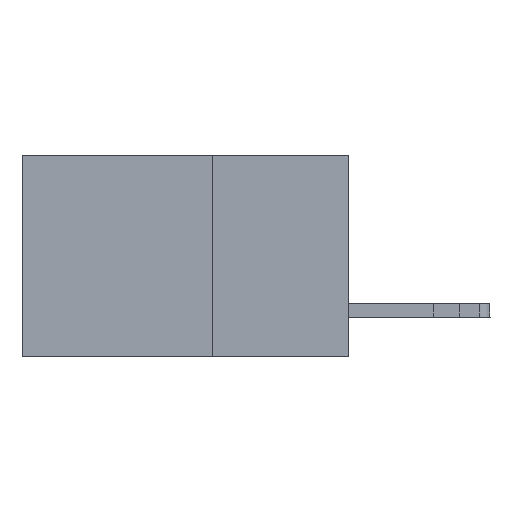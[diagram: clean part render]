
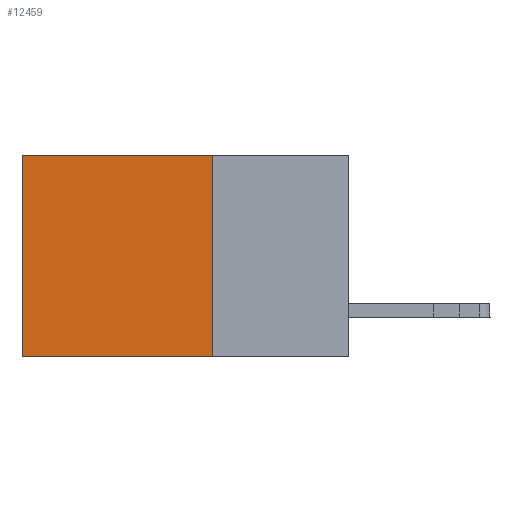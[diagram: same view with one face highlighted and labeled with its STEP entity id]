
A CAD part, left-side view. The second image highlights one B-rep face of the part: STEP entity #12459.
In plain terms, the highlighted planar face has unit normal (-1, 0, 0).
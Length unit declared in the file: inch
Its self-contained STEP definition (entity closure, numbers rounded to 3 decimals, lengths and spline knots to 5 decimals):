
#1073 = LINE ( 'NONE', #12287, #2677 ) ;
#2677 = VECTOR ( 'NONE', #16001, 39.37008 ) ;
#3276 = CARTESIAN_POINT ( 'NONE',  ( 0.298, 0.6, 0. ) ) ;
#3290 = CARTESIAN_POINT ( 'NONE',  ( 0.298, 0.25, 0. ) ) ;
#3370 = CARTESIAN_POINT ( 'NONE',  ( 0.298, 0.6, -0.37 ) ) ;
#4145 = VERTEX_POINT ( 'NONE', #3370 ) ;
#4219 = LINE ( 'NONE', #15275, #12650 ) ;
#4233 = LINE ( 'NONE', #16862, #18646 ) ;
#4337 = DIRECTION ( 'NONE',  ( 0., 1., 0. ) ) ;
#4975 = PLANE ( 'NONE',  #20713 ) ;
#5062 = DIRECTION ( 'NONE',  ( 0., 0., -1. ) ) ;
#5693 = EDGE_CURVE ( 'NONE', #22533, #14154, #4219, .T. ) ;
#7934 = CARTESIAN_POINT ( 'NONE',  ( 0.298, 0.25, 0. ) ) ;
#9949 = VECTOR ( 'NONE', #5062, 39.37008 ) ;
#10491 = CARTESIAN_POINT ( 'NONE',  ( 0.298, 0.25, 0. ) ) ;
#12287 = CARTESIAN_POINT ( 'NONE',  ( 0.298, 0.6, 0. ) ) ;
#12299 = LINE ( 'NONE', #10491, #9949 ) ;
#12459 = ADVANCED_FACE ( 'NONE', ( #23627 ), #4975, .F. ) ;
#12650 = VECTOR ( 'NONE', #4337, 39.37008 ) ;
#12944 = EDGE_CURVE ( 'NONE', #22533, #18994, #12299, .T. ) ;
#13648 = EDGE_LOOP ( 'NONE', ( #15808, #19429, #15370, #16116 ) ) ;
#14154 = VERTEX_POINT ( 'NONE', #3276 ) ;
#14368 = DIRECTION ( 'NONE',  ( 1., 0., 0. ) ) ;
#15275 = CARTESIAN_POINT ( 'NONE',  ( 0.298, 0.25, 0. ) ) ;
#15370 = ORIENTED_EDGE ( 'NONE', *, *, #12944, .F. ) ;
#15545 = EDGE_CURVE ( 'NONE', #18994, #4145, #4233, .T. ) ;
#15808 = ORIENTED_EDGE ( 'NONE', *, *, #22208, .T. ) ;
#16001 = DIRECTION ( 'NONE',  ( 0., 0., -1. ) ) ;
#16116 = ORIENTED_EDGE ( 'NONE', *, *, #5693, .T. ) ;
#16862 = CARTESIAN_POINT ( 'NONE',  ( 0.298, 0.25, -0.37 ) ) ;
#18646 = VECTOR ( 'NONE', #18668, 39.37008 ) ;
#18668 = DIRECTION ( 'NONE',  ( 0., 1., 0. ) ) ;
#18695 = CARTESIAN_POINT ( 'NONE',  ( 0.298, 0.25, -0.37 ) ) ;
#18994 = VERTEX_POINT ( 'NONE', #18695 ) ;
#19429 = ORIENTED_EDGE ( 'NONE', *, *, #15545, .F. ) ;
#20034 = DIRECTION ( 'NONE',  ( 0., 0., -1. ) ) ;
#20713 = AXIS2_PLACEMENT_3D ( 'NONE', #3290, #14368, #20034 ) ;
#22208 = EDGE_CURVE ( 'NONE', #14154, #4145, #1073, .T. ) ;
#22533 = VERTEX_POINT ( 'NONE', #7934 ) ;
#23627 = FACE_OUTER_BOUND ( 'NONE', #13648, .T. ) ;
